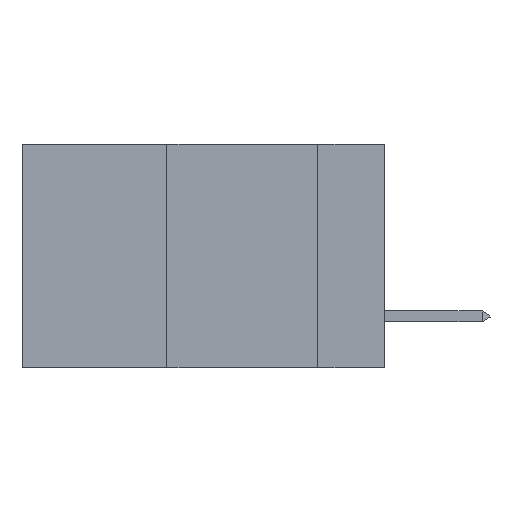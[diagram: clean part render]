
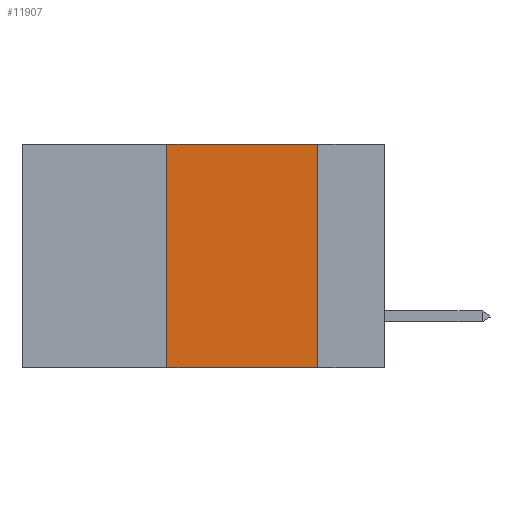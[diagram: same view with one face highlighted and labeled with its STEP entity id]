
A CAD part, left-side view. The second image highlights one B-rep face of the part: STEP entity #11907.
In plain terms, the highlighted planar face has unit normal (-1, 0, 0).
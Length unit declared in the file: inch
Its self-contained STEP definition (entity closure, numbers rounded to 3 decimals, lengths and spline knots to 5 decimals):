
#39 = CARTESIAN_POINT ( 'NONE',  ( 0., 0.6, -0.37 ) ) ;
#373 = ORIENTED_EDGE ( 'NONE', *, *, #2734, .F. ) ;
#492 = ORIENTED_EDGE ( 'NONE', *, *, #1424, .T. ) ;
#694 = EDGE_LOOP ( 'NONE', ( #20615, #785, #373, #492 ) ) ;
#785 = ORIENTED_EDGE ( 'NONE', *, *, #4885, .F. ) ;
#805 = DIRECTION ( 'NONE',  ( 0., 0., -1. ) ) ;
#1424 = EDGE_CURVE ( 'NONE', #22377, #15357, #11060, .T. ) ;
#1564 = VECTOR ( 'NONE', #4809, 39.37008 ) ;
#2146 = CARTESIAN_POINT ( 'NONE',  ( 0., 0.11, -0.37 ) ) ;
#2172 = DIRECTION ( 'NONE',  ( 1., 0., 0. ) ) ;
#2391 = VECTOR ( 'NONE', #8680, 39.37008 ) ;
#2613 = CARTESIAN_POINT ( 'NONE',  ( 0., 0.36, 0. ) ) ;
#2734 = EDGE_CURVE ( 'NONE', #22377, #14834, #17683, .T. ) ;
#3479 = AXIS2_PLACEMENT_3D ( 'NONE', #9757, #2172, #15564 ) ;
#4809 = DIRECTION ( 'NONE',  ( 0., -1., 0. ) ) ;
#4885 = EDGE_CURVE ( 'NONE', #14834, #6826, #22997, .T. ) ;
#6483 = CARTESIAN_POINT ( 'NONE',  ( 0., 0.11, 0. ) ) ;
#6826 = VERTEX_POINT ( 'NONE', #9630 ) ;
#8680 = DIRECTION ( 'NONE',  ( 0., 0., 1. ) ) ;
#9630 = CARTESIAN_POINT ( 'NONE',  ( 0., 0.11, 0. ) ) ;
#9757 = CARTESIAN_POINT ( 'NONE',  ( 0., 0.6, 0. ) ) ;
#11060 = LINE ( 'NONE', #39, #1564 ) ;
#11640 = PLANE ( 'NONE',  #3479 ) ;
#11907 = ADVANCED_FACE ( 'NONE', ( #17791 ), #11640, .F. ) ;
#12211 = CARTESIAN_POINT ( 'NONE',  ( 0., 0.6, 0. ) ) ;
#14834 = VERTEX_POINT ( 'NONE', #2613 ) ;
#15357 = VERTEX_POINT ( 'NONE', #2146 ) ;
#15541 = EDGE_CURVE ( 'NONE', #6826, #15357, #20423, .T. ) ;
#15564 = DIRECTION ( 'NONE',  ( 0., 0., -1. ) ) ;
#15583 = CARTESIAN_POINT ( 'NONE',  ( 0., 0.36, 0. ) ) ;
#17683 = LINE ( 'NONE', #15583, #2391 ) ;
#17791 = FACE_OUTER_BOUND ( 'NONE', #694, .T. ) ;
#18158 = VECTOR ( 'NONE', #21715, 39.37008 ) ;
#19258 = VECTOR ( 'NONE', #805, 39.37008 ) ;
#20062 = CARTESIAN_POINT ( 'NONE',  ( 0., 0.36, -0.37 ) ) ;
#20423 = LINE ( 'NONE', #6483, #19258 ) ;
#20615 = ORIENTED_EDGE ( 'NONE', *, *, #15541, .F. ) ;
#21715 = DIRECTION ( 'NONE',  ( 0., -1., 0. ) ) ;
#22377 = VERTEX_POINT ( 'NONE', #20062 ) ;
#22997 = LINE ( 'NONE', #12211, #18158 ) ;
